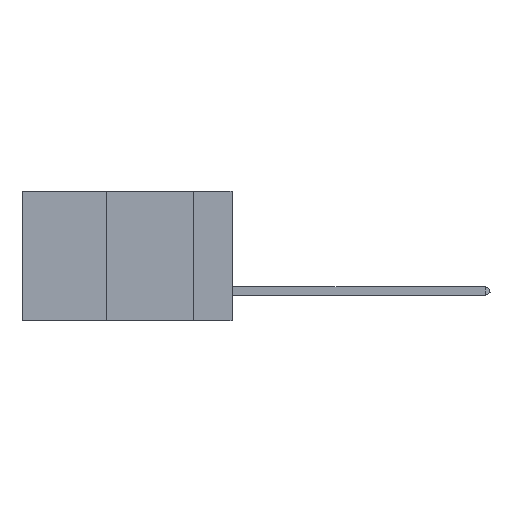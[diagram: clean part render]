
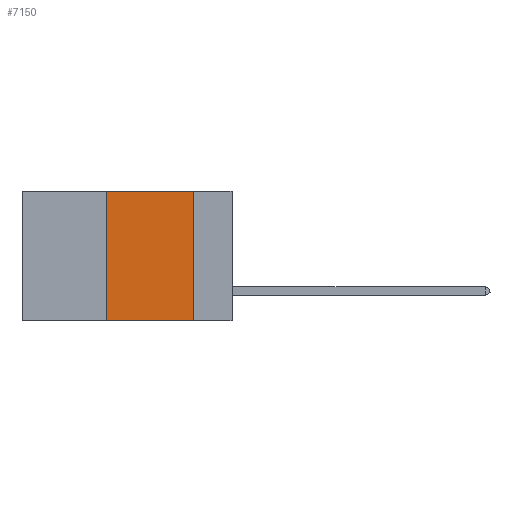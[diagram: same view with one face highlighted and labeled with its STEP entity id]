
A CAD part, left-side view. The second image highlights one B-rep face of the part: STEP entity #7150.
In plain terms, the highlighted planar face has unit normal (-1, 0, 0).
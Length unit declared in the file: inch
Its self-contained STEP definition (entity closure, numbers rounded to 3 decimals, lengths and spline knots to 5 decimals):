
#279 = PLANE ( 'NONE',  #3541 ) ;
#559 = CARTESIAN_POINT ( 'NONE',  ( 0., 0.36, -0.37 ) ) ;
#631 = LINE ( 'NONE', #12032, #28146 ) ;
#908 = CARTESIAN_POINT ( 'NONE',  ( 0., 0.11, -0.37 ) ) ;
#2712 = DIRECTION ( 'NONE',  ( 1., 0., 0. ) ) ;
#3541 = AXIS2_PLACEMENT_3D ( 'NONE', #19528, #2712, #36527 ) ;
#4851 = CARTESIAN_POINT ( 'NONE',  ( 0., 0.6, 0. ) ) ;
#4925 = CARTESIAN_POINT ( 'NONE',  ( 0., 0.36, 0. ) ) ;
#5400 = LINE ( 'NONE', #4851, #19227 ) ;
#7150 = ADVANCED_FACE ( 'NONE', ( #22886 ), #279, .F. ) ;
#8229 = VERTEX_POINT ( 'NONE', #559 ) ;
#8883 = CARTESIAN_POINT ( 'NONE',  ( 0., 0.6, -0.37 ) ) ;
#11084 = VECTOR ( 'NONE', #13875, 39.37008 ) ;
#11845 = VERTEX_POINT ( 'NONE', #25155 ) ;
#11973 = EDGE_CURVE ( 'NONE', #8229, #18398, #14865, .T. ) ;
#12032 = CARTESIAN_POINT ( 'NONE',  ( 0., 0.11, 0. ) ) ;
#13875 = DIRECTION ( 'NONE',  ( 0., 0., 1. ) ) ;
#14865 = LINE ( 'NONE', #8883, #27570 ) ;
#16786 = DIRECTION ( 'NONE',  ( 0., -1., 0. ) ) ;
#16855 = LINE ( 'NONE', #4925, #11084 ) ;
#17633 = EDGE_CURVE ( 'NONE', #8229, #17778, #16855, .T. ) ;
#17778 = VERTEX_POINT ( 'NONE', #26371 ) ;
#18398 = VERTEX_POINT ( 'NONE', #908 ) ;
#18582 = ORIENTED_EDGE ( 'NONE', *, *, #36109, .F. ) ;
#19227 = VECTOR ( 'NONE', #16786, 39.37008 ) ;
#19528 = CARTESIAN_POINT ( 'NONE',  ( 0., 0.6, 0. ) ) ;
#22886 = FACE_OUTER_BOUND ( 'NONE', #32302, .T. ) ;
#23413 = DIRECTION ( 'NONE',  ( 0., 0., -1. ) ) ;
#25155 = CARTESIAN_POINT ( 'NONE',  ( 0., 0.11, 0. ) ) ;
#25240 = EDGE_CURVE ( 'NONE', #11845, #18398, #631, .T. ) ;
#25277 = ORIENTED_EDGE ( 'NONE', *, *, #17633, .F. ) ;
#26371 = CARTESIAN_POINT ( 'NONE',  ( 0., 0.36, 0. ) ) ;
#27570 = VECTOR ( 'NONE', #31670, 39.37008 ) ;
#28146 = VECTOR ( 'NONE', #23413, 39.37008 ) ;
#31670 = DIRECTION ( 'NONE',  ( 0., -1., 0. ) ) ;
#32112 = ORIENTED_EDGE ( 'NONE', *, *, #11973, .T. ) ;
#32302 = EDGE_LOOP ( 'NONE', ( #35103, #18582, #25277, #32112 ) ) ;
#35103 = ORIENTED_EDGE ( 'NONE', *, *, #25240, .F. ) ;
#36109 = EDGE_CURVE ( 'NONE', #17778, #11845, #5400, .T. ) ;
#36527 = DIRECTION ( 'NONE',  ( 0., 0., -1. ) ) ;
